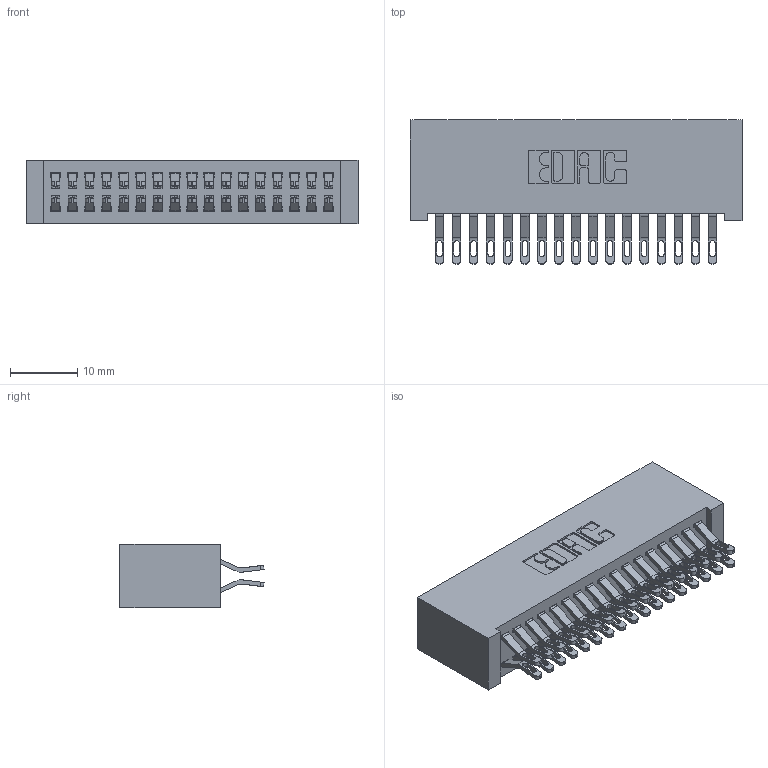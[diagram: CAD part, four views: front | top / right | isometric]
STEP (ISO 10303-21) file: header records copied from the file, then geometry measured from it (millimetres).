
FILE_DESCRIPTION (( 'STEP AP203' ), '1' );
FILE_NAME ('392-034-555-201.STEP', '2019-10-07T16:08:24', ( '' ), ( '' ), 'SwSTEP 2.0', 'SolidWorks 2016', '' );
FILE_SCHEMA (( 'CONFIG_CONTROL_DESIGN' ));
Length unit declared in the file: inch
Products named in the file (3): 342 Part_Lugless; 345-292-001_555 Tail; 392-034-555-201
Assembly tree (35 placements, depth 2):
  392-034-555-201
    342 Part_Lugless
    345-292-001_555 Tail  x34
Bounding box: 49.43 x 21.47 x 9.4 mm (x, y, z)
Volume: 4856.8 mm3; surface area: 8064.8 mm2
Topology: 35 solids, 35 shells, 2074 faces, 6497 edges, 4330 vertices
Faces by surface type: plane 1218, cylinder 856
Entity records: 14087 total; most frequent: CARTESIAN_POINT 2396, ORIENTED_EDGE 2302, DIRECTION 2055, EDGE_CURVE 1151, VECTOR 1011, LINE 1011, VERTEX_POINT 766, AXIS2_PLACEMENT_3D 522
